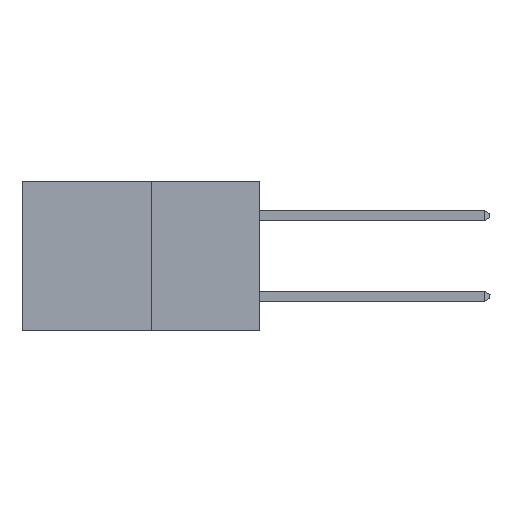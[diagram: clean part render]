
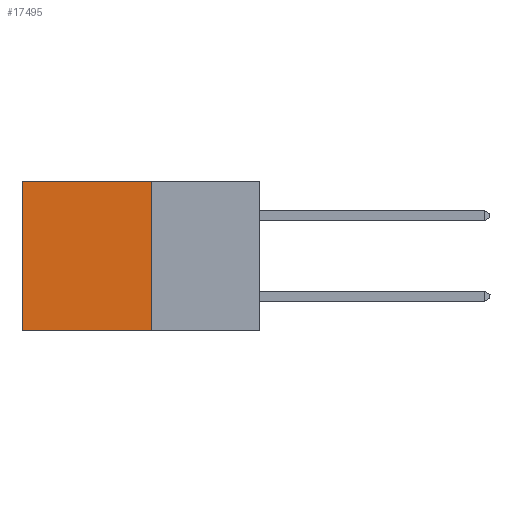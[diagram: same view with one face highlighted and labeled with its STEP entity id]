
A CAD part, left-side view. The second image highlights one B-rep face of the part: STEP entity #17495.
In plain terms, the highlighted planar face has unit normal (-1, 0, 0).
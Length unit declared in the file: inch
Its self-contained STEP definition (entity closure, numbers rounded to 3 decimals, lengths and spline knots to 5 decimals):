
#293 = EDGE_CURVE ( 'NONE', #7644, #16220, #13235, .T. ) ;
#1133 = FACE_OUTER_BOUND ( 'NONE', #4886, .T. ) ;
#2067 = CARTESIAN_POINT ( 'NONE',  ( 0.277, 0.59, -0.37 ) ) ;
#2403 = EDGE_CURVE ( 'NONE', #16220, #9672, #5131, .T. ) ;
#3765 = DIRECTION ( 'NONE',  ( 0., 1., 0. ) ) ;
#4356 = CARTESIAN_POINT ( 'NONE',  ( 0.277, 0.59, -0.37 ) ) ;
#4886 = EDGE_LOOP ( 'NONE', ( #13932, #15856, #16369, #21931 ) ) ;
#5131 = LINE ( 'NONE', #2067, #9278 ) ;
#5179 = VECTOR ( 'NONE', #3765, 39.37008 ) ;
#7205 = EDGE_CURVE ( 'NONE', #7644, #13741, #8759, .T. ) ;
#7644 = VERTEX_POINT ( 'NONE', #8722 ) ;
#8053 = DIRECTION ( 'NONE',  ( 0., 0., -1. ) ) ;
#8722 = CARTESIAN_POINT ( 'NONE',  ( 0.277, 0.27, 0. ) ) ;
#8759 = LINE ( 'NONE', #15301, #21667 ) ;
#8979 = DIRECTION ( 'NONE',  ( 1., 0., 0. ) ) ;
#9112 = VECTOR ( 'NONE', #15812, 39.37008 ) ;
#9278 = VECTOR ( 'NONE', #8053, 39.37008 ) ;
#9672 = VERTEX_POINT ( 'NONE', #4356 ) ;
#10407 = CARTESIAN_POINT ( 'NONE',  ( 0.277, 0.27, 0. ) ) ;
#10648 = CARTESIAN_POINT ( 'NONE',  ( 0.277, 0.59, 0. ) ) ;
#10676 = PLANE ( 'NONE',  #14576 ) ;
#12553 = CARTESIAN_POINT ( 'NONE',  ( 0.277, 0.27, -0.37 ) ) ;
#13235 = LINE ( 'NONE', #10407, #9112 ) ;
#13282 = CARTESIAN_POINT ( 'NONE',  ( 0.277, 0.27, -0.37 ) ) ;
#13741 = VERTEX_POINT ( 'NONE', #13282 ) ;
#13932 = ORIENTED_EDGE ( 'NONE', *, *, #2403, .T. ) ;
#14562 = LINE ( 'NONE', #12553, #5179 ) ;
#14576 = AXIS2_PLACEMENT_3D ( 'NONE', #19490, #8979, #21251 ) ;
#15301 = CARTESIAN_POINT ( 'NONE',  ( 0.277, 0.27, -0.37 ) ) ;
#15812 = DIRECTION ( 'NONE',  ( 0., 1., 0. ) ) ;
#15856 = ORIENTED_EDGE ( 'NONE', *, *, #21114, .F. ) ;
#16220 = VERTEX_POINT ( 'NONE', #10648 ) ;
#16369 = ORIENTED_EDGE ( 'NONE', *, *, #7205, .F. ) ;
#17495 = ADVANCED_FACE ( 'NONE', ( #1133 ), #10676, .F. ) ;
#17845 = DIRECTION ( 'NONE',  ( 0., 0., -1. ) ) ;
#19490 = CARTESIAN_POINT ( 'NONE',  ( 0.277, 0.27, -0.37 ) ) ;
#21114 = EDGE_CURVE ( 'NONE', #13741, #9672, #14562, .T. ) ;
#21251 = DIRECTION ( 'NONE',  ( 0., 0., -1. ) ) ;
#21667 = VECTOR ( 'NONE', #17845, 39.37008 ) ;
#21931 = ORIENTED_EDGE ( 'NONE', *, *, #293, .T. ) ;
